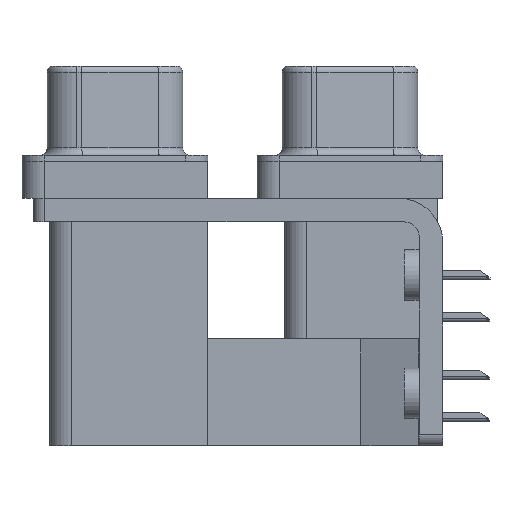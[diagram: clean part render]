
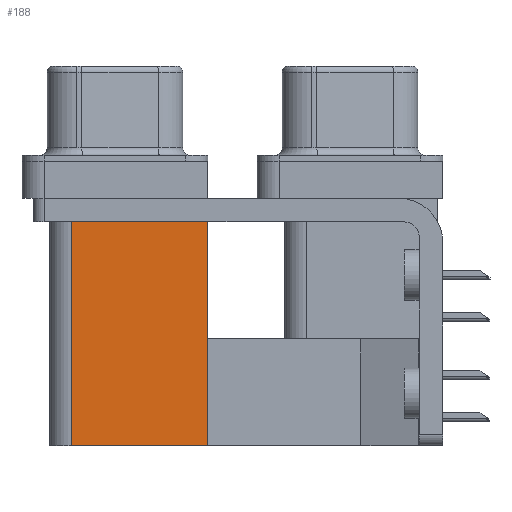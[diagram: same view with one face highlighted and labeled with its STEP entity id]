
A CAD part, left-side view. The second image highlights one B-rep face of the part: STEP entity #188.
In plain terms, the highlighted planar face has unit normal (-1, 0, 0).
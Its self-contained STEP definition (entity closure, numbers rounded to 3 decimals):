
#78 = CARTESIAN_POINT ( 'NONE',  ( 3.79, 9.6, -2.5 ) ) ;
#188 = ADVANCED_FACE ( 'NONE', ( #9774 ), #7925, .F. ) ;
#1266 = CARTESIAN_POINT ( 'NONE',  ( 3.79, 18.8, -2.5 ) ) ;
#2027 = CARTESIAN_POINT ( 'NONE',  ( 3.79, 9.6, -19.2 ) ) ;
#4124 = VERTEX_POINT ( 'NONE', #2027 ) ;
#4837 = CARTESIAN_POINT ( 'NONE',  ( 3.79, 9.6, -2.5 ) ) ;
#5784 = DIRECTION ( 'NONE',  ( 1., 0., 0. ) ) ;
#5954 = DIRECTION ( 'NONE',  ( 0., 1., 0. ) ) ;
#7925 = PLANE ( 'NONE',  #10850 ) ;
#8120 = DIRECTION ( 'NONE',  ( 0., 0., 1. ) ) ;
#8918 = EDGE_CURVE ( 'NONE', #4124, #21531, #14681, .T. ) ;
#9362 = VECTOR ( 'NONE', #5954, 1000. ) ;
#9774 = FACE_OUTER_BOUND ( 'NONE', #24339, .T. ) ;
#10358 = CARTESIAN_POINT ( 'NONE',  ( 3.79, 18.8, -19.2 ) ) ;
#10611 = ORIENTED_EDGE ( 'NONE', *, *, #8918, .T. ) ;
#10774 = DIRECTION ( 'NONE',  ( 0., 0., 1. ) ) ;
#10850 = AXIS2_PLACEMENT_3D ( 'NONE', #16926, #5784, #18785 ) ;
#12934 = LINE ( 'NONE', #16674, #9362 ) ;
#13265 = LINE ( 'NONE', #4837, #21831 ) ;
#13682 = VERTEX_POINT ( 'NONE', #1266 ) ;
#14681 = LINE ( 'NONE', #27689, #16991 ) ;
#16674 = CARTESIAN_POINT ( 'NONE',  ( 3.79, 9.6, -19.2 ) ) ;
#16926 = CARTESIAN_POINT ( 'NONE',  ( 3.79, 9.6, -19.2 ) ) ;
#16991 = VECTOR ( 'NONE', #8120, 1000. ) ;
#17541 = ORIENTED_EDGE ( 'NONE', *, *, #22547, .F. ) ;
#18785 = DIRECTION ( 'NONE',  ( 0., 0., -1. ) ) ;
#19836 = VECTOR ( 'NONE', #10774, 1000. ) ;
#21531 = VERTEX_POINT ( 'NONE', #78 ) ;
#21726 = EDGE_CURVE ( 'NONE', #27184, #13682, #23512, .T. ) ;
#21831 = VECTOR ( 'NONE', #22409, 1000. ) ;
#22409 = DIRECTION ( 'NONE',  ( 0., 1., 0. ) ) ;
#22547 = EDGE_CURVE ( 'NONE', #4124, #27184, #12934, .T. ) ;
#23512 = LINE ( 'NONE', #10358, #19836 ) ;
#24339 = EDGE_LOOP ( 'NONE', ( #26828, #25379, #17541, #10611 ) ) ;
#25379 = ORIENTED_EDGE ( 'NONE', *, *, #21726, .F. ) ;
#26449 = CARTESIAN_POINT ( 'NONE',  ( 3.79, 18.8, -19.2 ) ) ;
#26828 = ORIENTED_EDGE ( 'NONE', *, *, #27642, .T. ) ;
#27184 = VERTEX_POINT ( 'NONE', #26449 ) ;
#27642 = EDGE_CURVE ( 'NONE', #21531, #13682, #13265, .T. ) ;
#27689 = CARTESIAN_POINT ( 'NONE',  ( 3.79, 9.6, -19.2 ) ) ;
